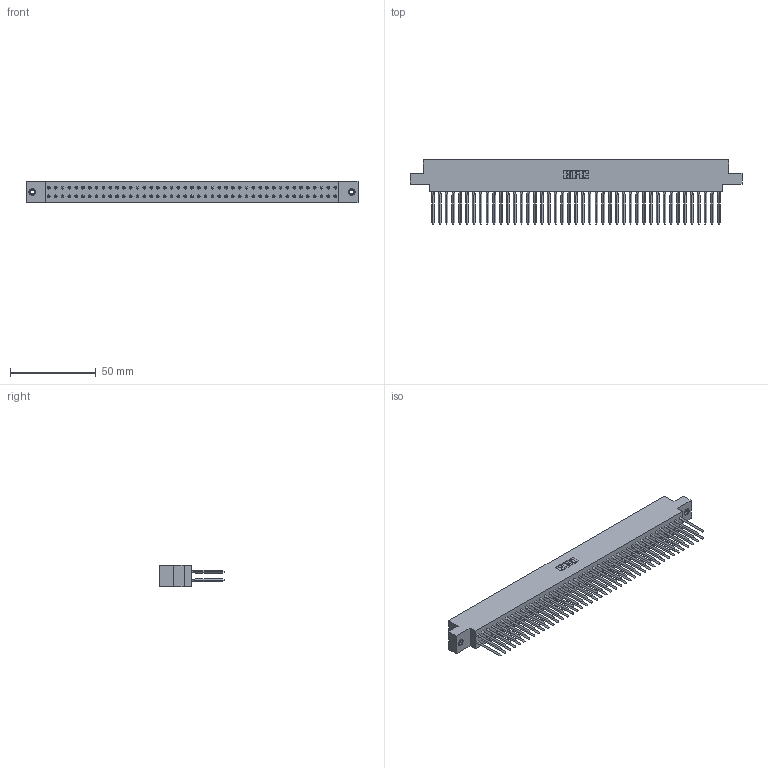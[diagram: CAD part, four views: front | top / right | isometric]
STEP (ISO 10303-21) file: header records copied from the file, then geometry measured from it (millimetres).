
FILE_DESCRIPTION (( 'STEP AP203' ), '1' );
FILE_NAME ('317-086-542-808.STEP', '2020-02-28T10:40:28', ( '' ), ( '' ), 'SwSTEP 2.0', 'SolidWorks 2016', '' );
FILE_SCHEMA (( 'CONFIG_CONTROL_DESIGN' ));
Length unit declared in the file: inch
Products named in the file (4): 345-250-001_345-250-003-102; 317-290-003_542; 317-086-542-808; 317 Part_.156 Dia - TI
Assembly tree (89 placements, depth 2):
  317-086-542-808
    317 Part_.156 Dia - TI
    317-290-003_542  x86
    345-250-001_345-250-003-102  x2
Bounding box: 193.09 x 37.34 x 12.7 mm (x, y, z)
Volume: 31643.1 mm3; surface area: 44057.2 mm2
Topology: 89 solids, 89 shells, 5064 faces, 14171 edges, 9038 vertices
Faces by surface type: plane 4046, cylinder 658, bspline 344, cone 12, torus 4
Entity records: 62220 total; most frequent: CARTESIAN_POINT 11076, ORIENTED_EDGE 10732, DIRECTION 9064, EDGE_CURVE 5366, LINE 5176, VECTOR 5176, VERTEX_POINT 3568, AXIS2_PLACEMENT_3D 1944
